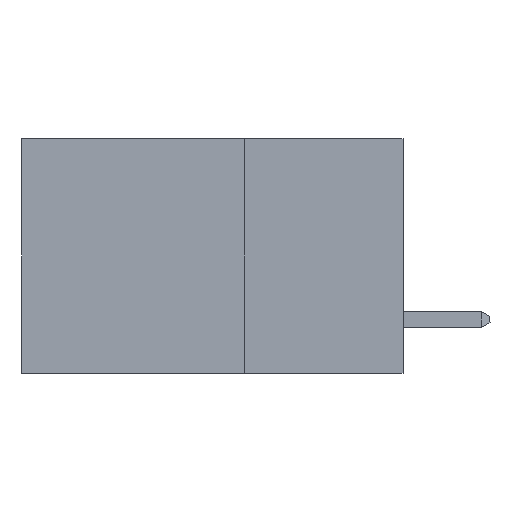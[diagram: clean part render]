
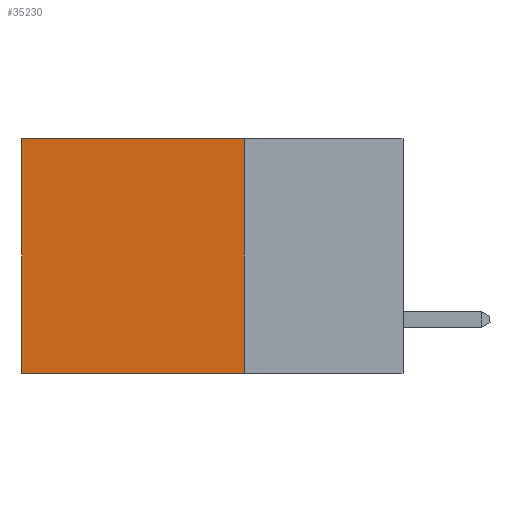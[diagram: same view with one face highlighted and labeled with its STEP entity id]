
A CAD part, left-side view. The second image highlights one B-rep face of the part: STEP entity #35230.
In plain terms, the highlighted planar face has unit normal (-1, 0, 0).
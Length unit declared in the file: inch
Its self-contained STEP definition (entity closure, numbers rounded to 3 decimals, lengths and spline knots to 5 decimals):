
#2498 = ORIENTED_EDGE ( 'NONE', *, *, #28576, .F. ) ;
#4635 = FACE_OUTER_BOUND ( 'NONE', #19376, .T. ) ;
#4717 = EDGE_CURVE ( 'NONE', #5527, #26370, #6909, .T. ) ;
#4902 = AXIS2_PLACEMENT_3D ( 'NONE', #13717, #5149, #25232 ) ;
#5149 = DIRECTION ( 'NONE',  ( 1., 0., 0. ) ) ;
#5527 = VERTEX_POINT ( 'NONE', #26284 ) ;
#5975 = VECTOR ( 'NONE', #31938, 39.37008 ) ;
#6866 = LINE ( 'NONE', #31818, #5975 ) ;
#6909 = LINE ( 'NONE', #13117, #12788 ) ;
#6965 = VECTOR ( 'NONE', #18990, 39.37008 ) ;
#10179 = DIRECTION ( 'NONE',  ( 0., 0., -1. ) ) ;
#11474 = VERTEX_POINT ( 'NONE', #27282 ) ;
#12080 = CARTESIAN_POINT ( 'NONE',  ( 0.2875, 0.6, 0. ) ) ;
#12558 = EDGE_CURVE ( 'NONE', #35404, #11474, #25371, .T. ) ;
#12788 = VECTOR ( 'NONE', #10179, 39.37008 ) ;
#13117 = CARTESIAN_POINT ( 'NONE',  ( 0.2875, 0.25, 0. ) ) ;
#13717 = CARTESIAN_POINT ( 'NONE',  ( 0.2875, 0.25, 0. ) ) ;
#13730 = LINE ( 'NONE', #36031, #6965 ) ;
#15944 = CARTESIAN_POINT ( 'NONE',  ( 0.2875, 0.25, -0.37 ) ) ;
#18990 = DIRECTION ( 'NONE',  ( 0., 1., 0. ) ) ;
#19376 = EDGE_LOOP ( 'NONE', ( #20496, #2498, #21356, #26150 ) ) ;
#20226 = CARTESIAN_POINT ( 'NONE',  ( 0.2875, 0.6, 0. ) ) ;
#20496 = ORIENTED_EDGE ( 'NONE', *, *, #12558, .T. ) ;
#20514 = EDGE_CURVE ( 'NONE', #5527, #35404, #13730, .T. ) ;
#21356 = ORIENTED_EDGE ( 'NONE', *, *, #4717, .F. ) ;
#22359 = PLANE ( 'NONE',  #4902 ) ;
#25232 = DIRECTION ( 'NONE',  ( 0., 0., -1. ) ) ;
#25371 = LINE ( 'NONE', #12080, #32940 ) ;
#26150 = ORIENTED_EDGE ( 'NONE', *, *, #20514, .T. ) ;
#26284 = CARTESIAN_POINT ( 'NONE',  ( 0.2875, 0.25, 0. ) ) ;
#26370 = VERTEX_POINT ( 'NONE', #15944 ) ;
#27282 = CARTESIAN_POINT ( 'NONE',  ( 0.2875, 0.6, -0.37 ) ) ;
#28576 = EDGE_CURVE ( 'NONE', #26370, #11474, #6866, .T. ) ;
#31818 = CARTESIAN_POINT ( 'NONE',  ( 0.2875, 0.25, -0.37 ) ) ;
#31938 = DIRECTION ( 'NONE',  ( 0., 1., 0. ) ) ;
#32083 = DIRECTION ( 'NONE',  ( 0., 0., -1. ) ) ;
#32940 = VECTOR ( 'NONE', #32083, 39.37008 ) ;
#35230 = ADVANCED_FACE ( 'NONE', ( #4635 ), #22359, .F. ) ;
#35404 = VERTEX_POINT ( 'NONE', #20226 ) ;
#36031 = CARTESIAN_POINT ( 'NONE',  ( 0.2875, 0.25, 0. ) ) ;
